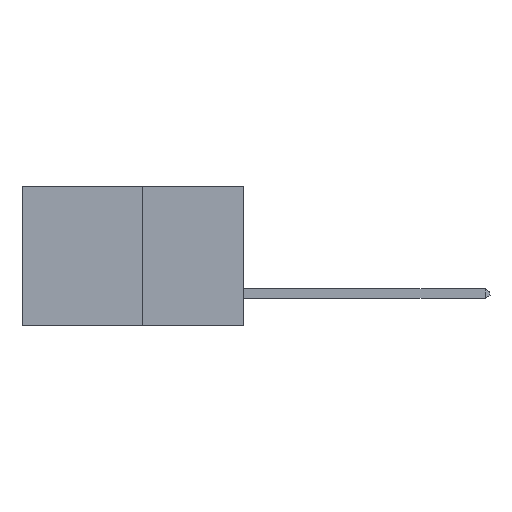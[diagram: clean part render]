
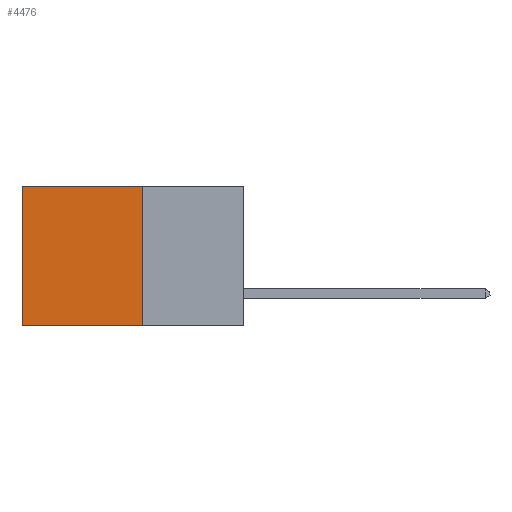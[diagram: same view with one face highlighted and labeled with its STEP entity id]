
A CAD part, left-side view. The second image highlights one B-rep face of the part: STEP entity #4476.
In plain terms, the highlighted planar face has unit normal (-1, 0, 0).
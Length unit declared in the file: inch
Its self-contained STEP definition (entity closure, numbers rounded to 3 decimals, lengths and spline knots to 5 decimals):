
#355 = CARTESIAN_POINT ( 'NONE',  ( 0.277, 0.27, -0.37 ) ) ;
#863 = VERTEX_POINT ( 'NONE', #355 ) ;
#906 = FACE_OUTER_BOUND ( 'NONE', #10221, .T. ) ;
#1700 = EDGE_CURVE ( 'NONE', #11529, #863, #5800, .T. ) ;
#1702 = VERTEX_POINT ( 'NONE', #8917 ) ;
#1786 = PLANE ( 'NONE',  #2517 ) ;
#1827 = DIRECTION ( 'NONE',  ( 1., 0., 0. ) ) ;
#1991 = ORIENTED_EDGE ( 'NONE', *, *, #1700, .F. ) ;
#2517 = AXIS2_PLACEMENT_3D ( 'NONE', #7945, #1827, #8979 ) ;
#2969 = ORIENTED_EDGE ( 'NONE', *, *, #4094, .T. ) ;
#3536 = CARTESIAN_POINT ( 'NONE',  ( 0.277, 0.59, 0. ) ) ;
#3835 = VECTOR ( 'NONE', #7301, 39.37008 ) ;
#4094 = EDGE_CURVE ( 'NONE', #11529, #10289, #8145, .T. ) ;
#4454 = CARTESIAN_POINT ( 'NONE',  ( 0.277, 0.27, 0. ) ) ;
#4476 = ADVANCED_FACE ( 'NONE', ( #906 ), #1786, .F. ) ;
#4908 = ORIENTED_EDGE ( 'NONE', *, *, #8061, .T. ) ;
#5436 = VECTOR ( 'NONE', #10224, 39.37008 ) ;
#5714 = DIRECTION ( 'NONE',  ( 0., 0., -1. ) ) ;
#5800 = LINE ( 'NONE', #8607, #10861 ) ;
#6250 = CARTESIAN_POINT ( 'NONE',  ( 0.277, 0.27, -0.37 ) ) ;
#6744 = LINE ( 'NONE', #6761, #9129 ) ;
#6761 = CARTESIAN_POINT ( 'NONE',  ( 0.277, 0.59, -0.37 ) ) ;
#7301 = DIRECTION ( 'NONE',  ( 0., 1., 0. ) ) ;
#7945 = CARTESIAN_POINT ( 'NONE',  ( 0.277, 0.27, -0.37 ) ) ;
#8061 = EDGE_CURVE ( 'NONE', #10289, #1702, #6744, .T. ) ;
#8145 = LINE ( 'NONE', #8217, #5436 ) ;
#8217 = CARTESIAN_POINT ( 'NONE',  ( 0.277, 0.27, 0. ) ) ;
#8297 = EDGE_CURVE ( 'NONE', #863, #1702, #8984, .T. ) ;
#8567 = DIRECTION ( 'NONE',  ( 0., 0., -1. ) ) ;
#8607 = CARTESIAN_POINT ( 'NONE',  ( 0.277, 0.27, -0.37 ) ) ;
#8917 = CARTESIAN_POINT ( 'NONE',  ( 0.277, 0.59, -0.37 ) ) ;
#8979 = DIRECTION ( 'NONE',  ( 0., 0., -1. ) ) ;
#8984 = LINE ( 'NONE', #6250, #3835 ) ;
#9129 = VECTOR ( 'NONE', #5714, 39.37008 ) ;
#10162 = ORIENTED_EDGE ( 'NONE', *, *, #8297, .F. ) ;
#10221 = EDGE_LOOP ( 'NONE', ( #4908, #10162, #1991, #2969 ) ) ;
#10224 = DIRECTION ( 'NONE',  ( 0., 1., 0. ) ) ;
#10289 = VERTEX_POINT ( 'NONE', #3536 ) ;
#10861 = VECTOR ( 'NONE', #8567, 39.37008 ) ;
#11529 = VERTEX_POINT ( 'NONE', #4454 ) ;
